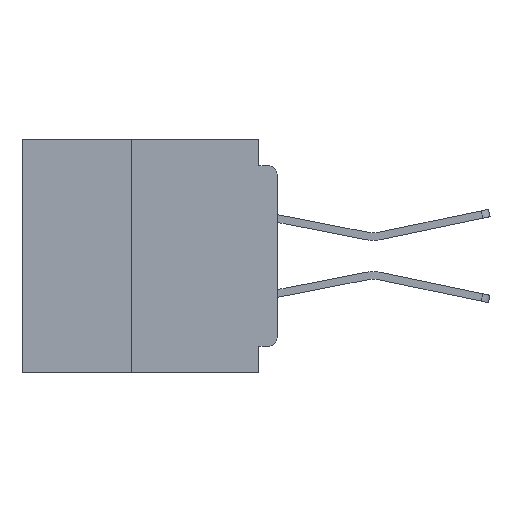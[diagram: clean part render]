
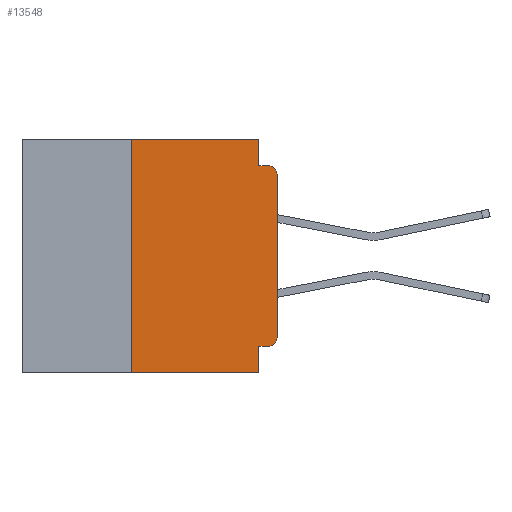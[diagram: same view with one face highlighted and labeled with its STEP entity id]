
A CAD part, left-side view. The second image highlights one B-rep face of the part: STEP entity #13548.
In plain terms, the highlighted planar face has unit normal (-1, 0, 0).
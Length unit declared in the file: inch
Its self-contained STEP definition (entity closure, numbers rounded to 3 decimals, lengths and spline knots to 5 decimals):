
#1219 = CARTESIAN_POINT ( 'NONE',  ( 0., 0.437, 0. ) ) ;
#2349 = DIRECTION ( 'NONE',  ( 0., -1., 0. ) ) ;
#2427 = ORIENTED_EDGE ( 'NONE', *, *, #42792, .F. ) ;
#2525 = DIRECTION ( 'NONE',  ( -1., 0., 0. ) ) ;
#3061 = AXIS2_PLACEMENT_3D ( 'NONE', #7172, #35449, #11266 ) ;
#3197 = LINE ( 'NONE', #5400, #12772 ) ;
#3575 = EDGE_CURVE ( 'NONE', #25377, #16156, #43007, .T. ) ;
#3707 = CARTESIAN_POINT ( 'NONE',  ( 0., 0.437, 0. ) ) ;
#5400 = CARTESIAN_POINT ( 'NONE',  ( 0., 0., 0. ) ) ;
#5898 = ORIENTED_EDGE ( 'NONE', *, *, #12173, .F. ) ;
#6191 = CARTESIAN_POINT ( 'NONE',  ( 0., 0., -0.34 ) ) ;
#6375 = ORIENTED_EDGE ( 'NONE', *, *, #24083, .T. ) ;
#6623 = VERTEX_POINT ( 'NONE', #19007 ) ;
#7172 = CARTESIAN_POINT ( 'NONE',  ( 0., 0.015, -0.34 ) ) ;
#8155 = VECTOR ( 'NONE', #48988, 39.37008 ) ;
#9188 = LINE ( 'NONE', #42591, #50594 ) ;
#10386 = FACE_OUTER_BOUND ( 'NONE', #43403, .T. ) ;
#10607 = LINE ( 'NONE', #3707, #20118 ) ;
#11006 = LINE ( 'NONE', #21023, #24347 ) ;
#11266 = DIRECTION ( 'NONE',  ( 0., 0., -1. ) ) ;
#12173 = EDGE_CURVE ( 'NONE', #16156, #47835, #20044, .T. ) ;
#12772 = VECTOR ( 'NONE', #29541, 39.37008 ) ;
#13308 = DIRECTION ( 'NONE',  ( 0., -1., 0. ) ) ;
#13539 = DIRECTION ( 'NONE',  ( 1., 0., 0. ) ) ;
#13548 = ADVANCED_FACE ( 'NONE', ( #10386 ), #49477, .F. ) ;
#14441 = VERTEX_POINT ( 'NONE', #49354 ) ;
#14937 = ORIENTED_EDGE ( 'NONE', *, *, #37122, .F. ) ;
#15334 = CARTESIAN_POINT ( 'NONE',  ( 0., 0.25, -0.4 ) ) ;
#15424 = CARTESIAN_POINT ( 'NONE',  ( 0., 0.031, -0.4 ) ) ;
#15491 = CARTESIAN_POINT ( 'NONE',  ( 0., 0., -0.06 ) ) ;
#16156 = VERTEX_POINT ( 'NONE', #36556 ) ;
#17858 = CARTESIAN_POINT ( 'NONE',  ( 0., 0.031, 0. ) ) ;
#19007 = CARTESIAN_POINT ( 'NONE',  ( 0., 0.25, 0. ) ) ;
#19295 = CIRCLE ( 'NONE', #3061, 0.015 ) ;
#20044 = LINE ( 'NONE', #37494, #29526 ) ;
#20118 = VECTOR ( 'NONE', #52010, 39.37008 ) ;
#20178 = VERTEX_POINT ( 'NONE', #6191 ) ;
#21023 = CARTESIAN_POINT ( 'NONE',  ( 0., 0., -0.355 ) ) ;
#21053 = CARTESIAN_POINT ( 'NONE',  ( 0., 0.25, -0.4 ) ) ;
#21159 = AXIS2_PLACEMENT_3D ( 'NONE', #26925, #2525, #30939 ) ;
#22229 = VERTEX_POINT ( 'NONE', #15424 ) ;
#22270 = ORIENTED_EDGE ( 'NONE', *, *, #28074, .F. ) ;
#22832 = LINE ( 'NONE', #26003, #42825 ) ;
#23470 = AXIS2_PLACEMENT_3D ( 'NONE', #1219, #13539, #41697 ) ;
#23554 = CARTESIAN_POINT ( 'NONE',  ( 0., 0.031, 0. ) ) ;
#24083 = EDGE_CURVE ( 'NONE', #14441, #20178, #19295, .T. ) ;
#24347 = VECTOR ( 'NONE', #44982, 39.37008 ) ;
#25377 = VERTEX_POINT ( 'NONE', #23554 ) ;
#26003 = CARTESIAN_POINT ( 'NONE',  ( 0., 0.031, -0.4 ) ) ;
#26890 = ORIENTED_EDGE ( 'NONE', *, *, #34848, .T. ) ;
#26925 = CARTESIAN_POINT ( 'NONE',  ( 0., 0.015, -0.06 ) ) ;
#28074 = EDGE_CURVE ( 'NONE', #6623, #25377, #10607, .T. ) ;
#29526 = VECTOR ( 'NONE', #13308, 39.37008 ) ;
#29541 = DIRECTION ( 'NONE',  ( 0., 0., 1. ) ) ;
#30939 = DIRECTION ( 'NONE',  ( 0., 0., -1. ) ) ;
#34212 = ORIENTED_EDGE ( 'NONE', *, *, #50391, .F. ) ;
#34848 = EDGE_CURVE ( 'NONE', #50772, #47835, #51009, .T. ) ;
#35449 = DIRECTION ( 'NONE',  ( -1., 0., 0. ) ) ;
#36556 = CARTESIAN_POINT ( 'NONE',  ( 0., 0.031, -0.045 ) ) ;
#37122 = EDGE_CURVE ( 'NONE', #44518, #22229, #22832, .T. ) ;
#37494 = CARTESIAN_POINT ( 'NONE',  ( 0., 0., -0.045 ) ) ;
#37764 = CARTESIAN_POINT ( 'NONE',  ( 0., 0.031, -0.355 ) ) ;
#37926 = DIRECTION ( 'NONE',  ( 0., 0., -1. ) ) ;
#38248 = ORIENTED_EDGE ( 'NONE', *, *, #3575, .F. ) ;
#39097 = LINE ( 'NONE', #21053, #8155 ) ;
#39814 = EDGE_CURVE ( 'NONE', #44785, #22229, #9188, .T. ) ;
#41159 = ORIENTED_EDGE ( 'NONE', *, *, #39814, .T. ) ;
#41697 = DIRECTION ( 'NONE',  ( 0., 0., -1. ) ) ;
#41778 = VECTOR ( 'NONE', #37926, 39.37008 ) ;
#42591 = CARTESIAN_POINT ( 'NONE',  ( 0., 0.437, -0.4 ) ) ;
#42792 = EDGE_CURVE ( 'NONE', #14441, #44518, #11006, .T. ) ;
#42825 = VECTOR ( 'NONE', #49831, 39.37008 ) ;
#43007 = LINE ( 'NONE', #17858, #41778 ) ;
#43403 = EDGE_LOOP ( 'NONE', ( #52011, #26890, #5898, #38248, #22270, #34212, #41159, #14937, #2427, #6375 ) ) ;
#44478 = EDGE_CURVE ( 'NONE', #20178, #50772, #3197, .T. ) ;
#44518 = VERTEX_POINT ( 'NONE', #37764 ) ;
#44785 = VERTEX_POINT ( 'NONE', #15334 ) ;
#44982 = DIRECTION ( 'NONE',  ( 0., 1., 0. ) ) ;
#47835 = VERTEX_POINT ( 'NONE', #50185 ) ;
#48988 = DIRECTION ( 'NONE',  ( 0., 0., 1. ) ) ;
#49354 = CARTESIAN_POINT ( 'NONE',  ( 0., 0.015, -0.355 ) ) ;
#49477 = PLANE ( 'NONE',  #23470 ) ;
#49831 = DIRECTION ( 'NONE',  ( 0., 0., -1. ) ) ;
#50185 = CARTESIAN_POINT ( 'NONE',  ( 0., 0.015, -0.045 ) ) ;
#50391 = EDGE_CURVE ( 'NONE', #44785, #6623, #39097, .T. ) ;
#50594 = VECTOR ( 'NONE', #2349, 39.37008 ) ;
#50772 = VERTEX_POINT ( 'NONE', #15491 ) ;
#51009 = CIRCLE ( 'NONE', #21159, 0.015 ) ;
#52010 = DIRECTION ( 'NONE',  ( 0., -1., 0. ) ) ;
#52011 = ORIENTED_EDGE ( 'NONE', *, *, #44478, .T. ) ;
